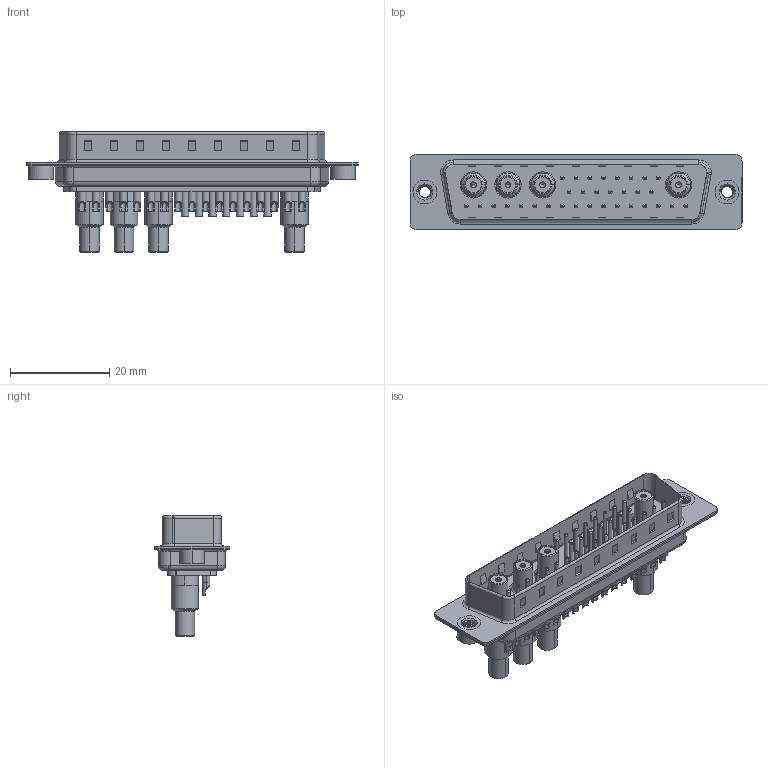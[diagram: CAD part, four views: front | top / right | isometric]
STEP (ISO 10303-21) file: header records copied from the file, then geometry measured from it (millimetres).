
FILE_DESCRIPTION (( 'STEP AP203' ), '1' );
FILE_NAME ('627-36W4622-5TA.STEP', '2019-06-19T07:12:43', ( '' ), ( '' ), 'SwSTEP 2.0', 'SolidWorks 2016', '' );
FILE_SCHEMA (( 'CONFIG_CONTROL_DESIGN' ));
Length unit declared in the file: millimetre
Products named in the file (15): 627Combo Contact Row 1_22; 627Combo Shell Rear_50 Contacts; 627Combo Contact Row 2_22L; 627Combo Shell Front_50 Contacts; 627Combo Contact Row 3_22; Insulator Socket; 627Combo Threaded Rivet_A; 627-36W4622-5TA; Insulator Socket 2; Co-Ax Jack_Solder Cup Tail; Locking Collar; Socket_Solder Cup; Solder Cover; Co-Ax Jack Assy_SC; 627Combo Housing_36W4
Assembly tree (47 placements, depth 3):
  627-36W4622-5TA
    627Combo Housing_36W4
    627Combo Shell Rear_50 Contacts
    627Combo Shell Front_50 Contacts
    627Combo Threaded Rivet_A  x2
    Co-Ax Jack Assy_SC  x4
      Co-Ax Jack_Solder Cup Tail
      Insulator Socket
      Insulator Socket 2
      Locking Collar
      Socket_Solder Cup
      Solder Cover
    627Combo Contact Row 1_22  x8
    627Combo Contact Row 2_22L  x7
    627Combo Contact Row 3_22  x17
Bounding box: 67 x 15.3 x 24.3 mm (x, y, z)
Volume: 5103.1 mm3; surface area: 14368.3 mm2
Topology: 61 solids, 61 shells, 2114 faces, 4895 edges, 2998 vertices
Faces by surface type: cylinder 911, plane 651, torus 386, cone 152, bspline 14
Entity records: 29984 total; most frequent: CARTESIAN_POINT 6397, DIRECTION 4748, ORIENTED_EDGE 4120, EDGE_CURVE 2060, AXIS2_PLACEMENT_3D 1867, VERTEX_POINT 1313, EDGE_LOOP 1091, VECTOR 1014
